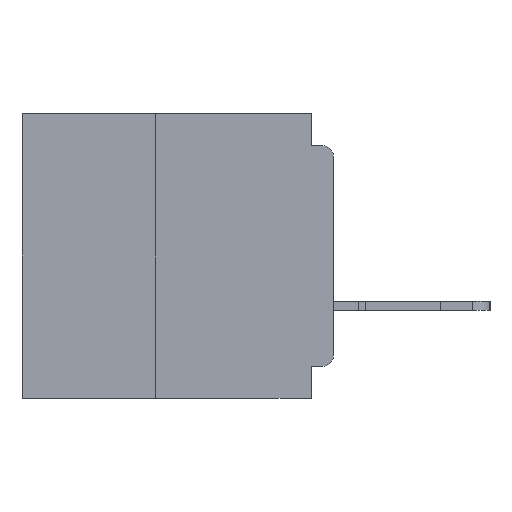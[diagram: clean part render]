
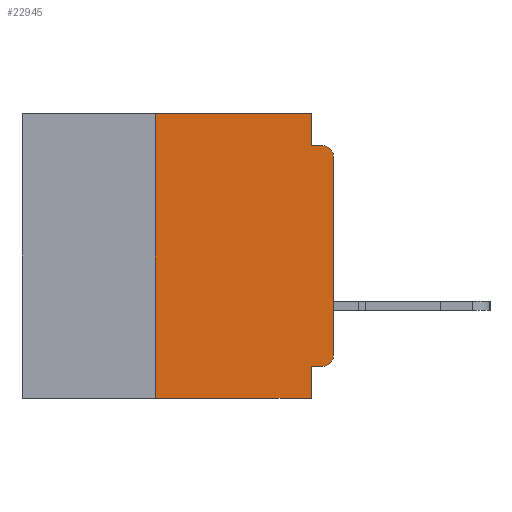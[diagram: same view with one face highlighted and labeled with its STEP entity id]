
A CAD part, left-side view. The second image highlights one B-rep face of the part: STEP entity #22945.
In plain terms, the highlighted planar face has unit normal (-1, 0, 0).
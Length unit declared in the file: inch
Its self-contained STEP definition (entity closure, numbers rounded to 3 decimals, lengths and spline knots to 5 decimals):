
#1453 = ORIENTED_EDGE ( 'NONE', *, *, #4389, .F. ) ;
#2961 = DIRECTION ( 'NONE',  ( 0., 0., -1. ) ) ;
#2988 = VERTEX_POINT ( 'NONE', #42713 ) ;
#3997 = CARTESIAN_POINT ( 'NONE',  ( 0., 0.031, -0.4 ) ) ;
#4092 = ORIENTED_EDGE ( 'NONE', *, *, #38679, .F. ) ;
#4389 = EDGE_CURVE ( 'NONE', #41358, #54752, #7160, .T. ) ;
#4491 = EDGE_CURVE ( 'NONE', #10981, #27402, #34191, .T. ) ;
#4861 = VERTEX_POINT ( 'NONE', #40092 ) ;
#5182 = VECTOR ( 'NONE', #5928, 39.37008 ) ;
#5288 = EDGE_CURVE ( 'NONE', #27402, #53466, #42443, .T. ) ;
#5928 = DIRECTION ( 'NONE',  ( 0., -1., 0. ) ) ;
#5981 = LINE ( 'NONE', #16424, #54034 ) ;
#6185 = PLANE ( 'NONE',  #18264 ) ;
#6322 = CARTESIAN_POINT ( 'NONE',  ( 0., 0.25, -0.4 ) ) ;
#7160 = LINE ( 'NONE', #3997, #39996 ) ;
#8297 = EDGE_CURVE ( 'NONE', #13244, #41358, #11593, .T. ) ;
#9475 = EDGE_CURVE ( 'NONE', #53466, #4861, #55657, .T. ) ;
#10981 = VERTEX_POINT ( 'NONE', #6322 ) ;
#11074 = EDGE_CURVE ( 'NONE', #41721, #34701, #5981, .T. ) ;
#11435 = LINE ( 'NONE', #21061, #59278 ) ;
#11593 = LINE ( 'NONE', #60077, #34904 ) ;
#11719 = DIRECTION ( 'NONE',  ( 0., 0., 1. ) ) ;
#13244 = VERTEX_POINT ( 'NONE', #40886 ) ;
#13392 = EDGE_CURVE ( 'NONE', #34701, #2988, #39423, .T. ) ;
#14027 = CARTESIAN_POINT ( 'NONE',  ( 0., 0.015, -0.06 ) ) ;
#14298 = DIRECTION ( 'NONE',  ( 0., 0., 1. ) ) ;
#15099 = LINE ( 'NONE', #57249, #50697 ) ;
#16424 = CARTESIAN_POINT ( 'NONE',  ( 0., 0., 0. ) ) ;
#18264 = AXIS2_PLACEMENT_3D ( 'NONE', #25049, #57404, #29746 ) ;
#18742 = DIRECTION ( 'NONE',  ( 0., 0., -1. ) ) ;
#19238 = DIRECTION ( 'NONE',  ( 0., 0., -1. ) ) ;
#19483 = CARTESIAN_POINT ( 'NONE',  ( 0., 0.031, 0. ) ) ;
#21061 = CARTESIAN_POINT ( 'NONE',  ( 0., 0., -0.045 ) ) ;
#22945 = ADVANCED_FACE ( 'NONE', ( #34582 ), #6185, .F. ) ;
#23480 = CARTESIAN_POINT ( 'NONE',  ( 0., 0.25, -0.4 ) ) ;
#23589 = ORIENTED_EDGE ( 'NONE', *, *, #36519, .T. ) ;
#25049 = CARTESIAN_POINT ( 'NONE',  ( 0., 0.437, 0. ) ) ;
#25324 = ORIENTED_EDGE ( 'NONE', *, *, #9475, .F. ) ;
#25332 = ORIENTED_EDGE ( 'NONE', *, *, #11074, .T. ) ;
#25721 = DIRECTION ( 'NONE',  ( 0., -1., 0. ) ) ;
#25779 = ORIENTED_EDGE ( 'NONE', *, *, #13392, .T. ) ;
#27362 = ORIENTED_EDGE ( 'NONE', *, *, #5288, .F. ) ;
#27402 = VERTEX_POINT ( 'NONE', #42480 ) ;
#29119 = ORIENTED_EDGE ( 'NONE', *, *, #4491, .F. ) ;
#29746 = DIRECTION ( 'NONE',  ( 0., 0., -1. ) ) ;
#31041 = DIRECTION ( 'NONE',  ( -1., 0., 0. ) ) ;
#31544 = ORIENTED_EDGE ( 'NONE', *, *, #45662, .T. ) ;
#32131 = CIRCLE ( 'NONE', #57232, 0.015 ) ;
#34191 = LINE ( 'NONE', #23480, #45048 ) ;
#34264 = DIRECTION ( 'NONE',  ( 0., -1., 0. ) ) ;
#34582 = FACE_OUTER_BOUND ( 'NONE', #40785, .T. ) ;
#34623 = AXIS2_PLACEMENT_3D ( 'NONE', #14027, #46529, #18742 ) ;
#34701 = VERTEX_POINT ( 'NONE', #55387 ) ;
#34904 = VECTOR ( 'NONE', #55444, 39.37008 ) ;
#36519 = EDGE_CURVE ( 'NONE', #13244, #41721, #32131, .T. ) ;
#37033 = CARTESIAN_POINT ( 'NONE',  ( 0., 0., -0.34 ) ) ;
#38638 = CARTESIAN_POINT ( 'NONE',  ( 0., 0.437, 0. ) ) ;
#38669 = ORIENTED_EDGE ( 'NONE', *, *, #8297, .F. ) ;
#38679 = EDGE_CURVE ( 'NONE', #4861, #2988, #11435, .T. ) ;
#39423 = CIRCLE ( 'NONE', #34623, 0.015 ) ;
#39996 = VECTOR ( 'NONE', #41339, 39.37008 ) ;
#40092 = CARTESIAN_POINT ( 'NONE',  ( 0., 0.031, -0.045 ) ) ;
#40785 = EDGE_LOOP ( 'NONE', ( #25332, #25779, #4092, #25324, #27362, #29119, #31544, #1453, #38669, #23589 ) ) ;
#40886 = CARTESIAN_POINT ( 'NONE',  ( 0., 0.015, -0.355 ) ) ;
#41339 = DIRECTION ( 'NONE',  ( 0., 0., -1. ) ) ;
#41358 = VERTEX_POINT ( 'NONE', #57241 ) ;
#41721 = VERTEX_POINT ( 'NONE', #37033 ) ;
#42443 = LINE ( 'NONE', #38638, #5182 ) ;
#42480 = CARTESIAN_POINT ( 'NONE',  ( 0., 0.25, 0. ) ) ;
#42713 = CARTESIAN_POINT ( 'NONE',  ( 0., 0.015, -0.045 ) ) ;
#45048 = VECTOR ( 'NONE', #14298, 39.37008 ) ;
#45662 = EDGE_CURVE ( 'NONE', #10981, #54752, #15099, .T. ) ;
#46529 = DIRECTION ( 'NONE',  ( -1., 0., 0. ) ) ;
#50697 = VECTOR ( 'NONE', #34264, 39.37008 ) ;
#51653 = CARTESIAN_POINT ( 'NONE',  ( 0., 0.031, 0. ) ) ;
#53466 = VERTEX_POINT ( 'NONE', #19483 ) ;
#54034 = VECTOR ( 'NONE', #11719, 39.37008 ) ;
#54243 = VECTOR ( 'NONE', #19238, 39.37008 ) ;
#54752 = VERTEX_POINT ( 'NONE', #55926 ) ;
#55387 = CARTESIAN_POINT ( 'NONE',  ( 0., 0., -0.06 ) ) ;
#55444 = DIRECTION ( 'NONE',  ( 0., 1., 0. ) ) ;
#55657 = LINE ( 'NONE', #51653, #54243 ) ;
#55926 = CARTESIAN_POINT ( 'NONE',  ( 0., 0.031, -0.4 ) ) ;
#57232 = AXIS2_PLACEMENT_3D ( 'NONE', #58683, #31041, #2961 ) ;
#57241 = CARTESIAN_POINT ( 'NONE',  ( 0., 0.031, -0.355 ) ) ;
#57249 = CARTESIAN_POINT ( 'NONE',  ( 0., 0.437, -0.4 ) ) ;
#57404 = DIRECTION ( 'NONE',  ( 1., 0., 0. ) ) ;
#58683 = CARTESIAN_POINT ( 'NONE',  ( 0., 0.015, -0.34 ) ) ;
#59278 = VECTOR ( 'NONE', #25721, 39.37008 ) ;
#60077 = CARTESIAN_POINT ( 'NONE',  ( 0., 0., -0.355 ) ) ;
